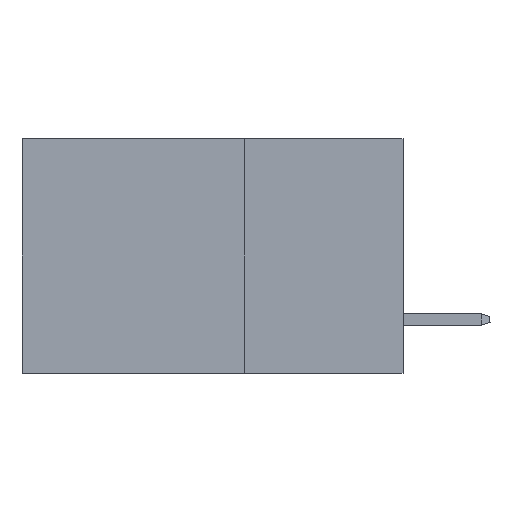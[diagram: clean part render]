
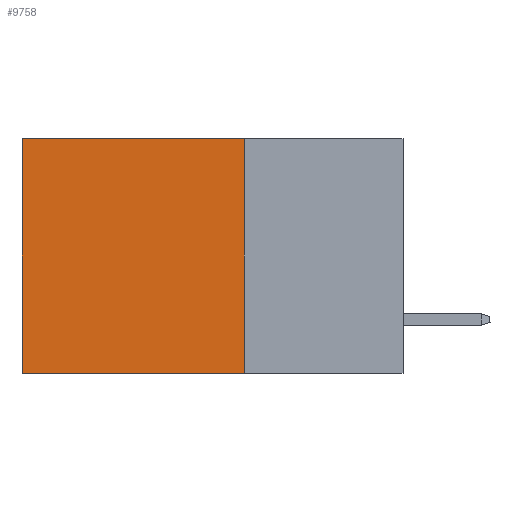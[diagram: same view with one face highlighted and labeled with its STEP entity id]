
A CAD part, left-side view. The second image highlights one B-rep face of the part: STEP entity #9758.
In plain terms, the highlighted planar face has unit normal (-1, 0, 0).
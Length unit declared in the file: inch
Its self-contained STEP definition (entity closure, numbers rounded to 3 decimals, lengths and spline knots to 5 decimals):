
#149 = AXIS2_PLACEMENT_3D ( 'NONE', #10647, #8727, #6703 ) ;
#1434 = CARTESIAN_POINT ( 'NONE',  ( 0.2875, 0.25, -0.37 ) ) ;
#3519 = VECTOR ( 'NONE', #13035, 39.37008 ) ;
#3842 = CARTESIAN_POINT ( 'NONE',  ( 0.2875, 0.6, 0. ) ) ;
#4544 = EDGE_LOOP ( 'NONE', ( #18908, #9223, #20994, #18914 ) ) ;
#5192 = LINE ( 'NONE', #5466, #7408 ) ;
#5466 = CARTESIAN_POINT ( 'NONE',  ( 0.2875, 0.25, 0. ) ) ;
#6703 = DIRECTION ( 'NONE',  ( 0., 0., -1. ) ) ;
#7286 = EDGE_CURVE ( 'NONE', #16145, #10714, #5192, .T. ) ;
#7408 = VECTOR ( 'NONE', #23995, 39.37008 ) ;
#7568 = VECTOR ( 'NONE', #8716, 39.37008 ) ;
#8587 = CARTESIAN_POINT ( 'NONE',  ( 0.2875, 0.6, 0. ) ) ;
#8716 = DIRECTION ( 'NONE',  ( 0., 0., -1. ) ) ;
#8727 = DIRECTION ( 'NONE',  ( 1., 0., 0. ) ) ;
#9096 = LINE ( 'NONE', #23317, #3519 ) ;
#9152 = DIRECTION ( 'NONE',  ( 0., 1., 0. ) ) ;
#9223 = ORIENTED_EDGE ( 'NONE', *, *, #16130, .F. ) ;
#9758 = ADVANCED_FACE ( 'NONE', ( #17274 ), #23212, .F. ) ;
#10647 = CARTESIAN_POINT ( 'NONE',  ( 0.2875, 0.25, 0. ) ) ;
#10714 = VERTEX_POINT ( 'NONE', #1434 ) ;
#11179 = CARTESIAN_POINT ( 'NONE',  ( 0.2875, 0.6, -0.37 ) ) ;
#12384 = VERTEX_POINT ( 'NONE', #11179 ) ;
#12744 = EDGE_CURVE ( 'NONE', #16145, #21786, #25519, .T. ) ;
#13035 = DIRECTION ( 'NONE',  ( 0., 1., 0. ) ) ;
#16130 = EDGE_CURVE ( 'NONE', #10714, #12384, #9096, .T. ) ;
#16145 = VERTEX_POINT ( 'NONE', #21824 ) ;
#17274 = FACE_OUTER_BOUND ( 'NONE', #4544, .T. ) ;
#18908 = ORIENTED_EDGE ( 'NONE', *, *, #21524, .T. ) ;
#18914 = ORIENTED_EDGE ( 'NONE', *, *, #12744, .T. ) ;
#19719 = VECTOR ( 'NONE', #9152, 39.37008 ) ;
#20994 = ORIENTED_EDGE ( 'NONE', *, *, #7286, .F. ) ;
#21428 = LINE ( 'NONE', #8587, #7568 ) ;
#21524 = EDGE_CURVE ( 'NONE', #21786, #12384, #21428, .T. ) ;
#21786 = VERTEX_POINT ( 'NONE', #3842 ) ;
#21824 = CARTESIAN_POINT ( 'NONE',  ( 0.2875, 0.25, 0. ) ) ;
#23212 = PLANE ( 'NONE',  #149 ) ;
#23317 = CARTESIAN_POINT ( 'NONE',  ( 0.2875, 0.25, -0.37 ) ) ;
#23995 = DIRECTION ( 'NONE',  ( 0., 0., -1. ) ) ;
#25382 = CARTESIAN_POINT ( 'NONE',  ( 0.2875, 0.25, 0. ) ) ;
#25519 = LINE ( 'NONE', #25382, #19719 ) ;
